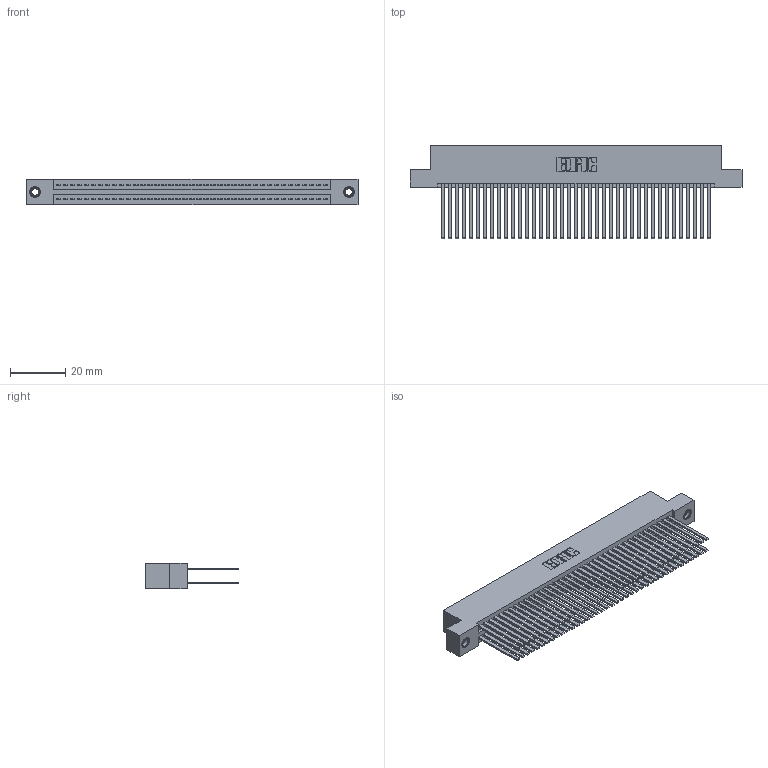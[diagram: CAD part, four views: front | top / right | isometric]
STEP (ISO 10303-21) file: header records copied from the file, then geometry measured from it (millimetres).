
FILE_DESCRIPTION (( 'STEP AP203' ), '1' );
FILE_NAME ('395-078-544-207.STEP', '2018-11-28T01:04:08', ( '' ), ( '' ), 'SwSTEP 2.0', 'SolidWorks 2016', '' );
FILE_SCHEMA (( 'CONFIG_CONTROL_DESIGN' ));
Length unit declared in the file: inch
Products named in the file (4): 395-078-544-207; 345 Part_Flush Mounting Lugs - 0.156 Dia-TI; 345-250-001_345-250-005-103; 345-292-001_345-293-144
Assembly tree (81 placements, depth 2):
  395-078-544-207
    345 Part_Flush Mounting Lugs - 0.156 Dia-TI
    345-292-001_345-293-144  x78
    345-250-001_345-250-005-103  x2
Bounding box: 120.27 x 33.96 x 9.4 mm (x, y, z)
Volume: 12735.1 mm3; surface area: 21999.1 mm2
Topology: 81 solids, 81 shells, 3618 faces, 10695 edges, 7018 vertices
Faces by surface type: plane 2374, cylinder 1228, cone 12, torus 4
Entity records: 32006 total; most frequent: CARTESIAN_POINT 5347, ORIENTED_EDGE 5274, DIRECTION 4743, EDGE_CURVE 2637, LINE 2333, VECTOR 2333, VERTEX_POINT 1752, AXIS2_PLACEMENT_3D 1205
